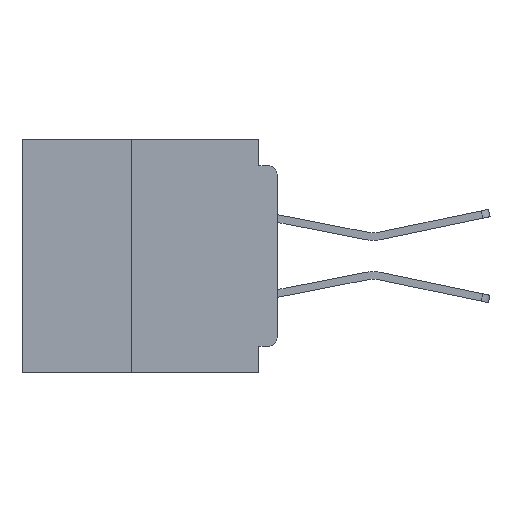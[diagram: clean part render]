
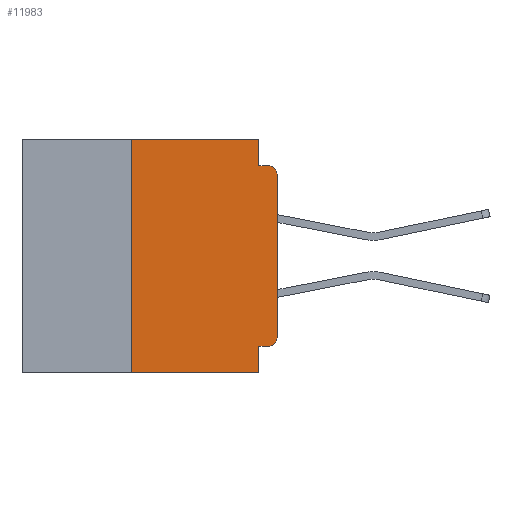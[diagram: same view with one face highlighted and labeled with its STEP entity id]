
A CAD part, left-side view. The second image highlights one B-rep face of the part: STEP entity #11983.
In plain terms, the highlighted planar face has unit normal (-1, 0, 0).
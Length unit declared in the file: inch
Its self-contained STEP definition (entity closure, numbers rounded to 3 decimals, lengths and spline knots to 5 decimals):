
#586 = DIRECTION ( 'NONE',  ( 0., 0., 1. ) ) ;
#776 = CARTESIAN_POINT ( 'NONE',  ( 0., 0.437, 0. ) ) ;
#959 = CARTESIAN_POINT ( 'NONE',  ( 0., 0.031, -0.4 ) ) ;
#1119 = LINE ( 'NONE', #18696, #9593 ) ;
#1357 = DIRECTION ( 'NONE',  ( 0., 0., -1. ) ) ;
#1956 = LINE ( 'NONE', #25080, #34847 ) ;
#2058 = LINE ( 'NONE', #19631, #9554 ) ;
#2086 = DIRECTION ( 'NONE',  ( -1., 0., 0. ) ) ;
#2098 = CARTESIAN_POINT ( 'NONE',  ( 0., 0.015, -0.06 ) ) ;
#2167 = CARTESIAN_POINT ( 'NONE',  ( 0., 0.015, -0.34 ) ) ;
#3313 = LINE ( 'NONE', #27133, #19255 ) ;
#3982 = PLANE ( 'NONE',  #41075 ) ;
#5369 = DIRECTION ( 'NONE',  ( 0., 0., -1. ) ) ;
#5922 = DIRECTION ( 'NONE',  ( 0., -1., 0. ) ) ;
#5979 = EDGE_CURVE ( 'NONE', #35043, #15358, #17767, .T. ) ;
#7226 = DIRECTION ( 'NONE',  ( 0., 0., -1. ) ) ;
#7338 = FACE_OUTER_BOUND ( 'NONE', #20604, .T. ) ;
#8306 = VERTEX_POINT ( 'NONE', #17071 ) ;
#8848 = ORIENTED_EDGE ( 'NONE', *, *, #27979, .F. ) ;
#9200 = DIRECTION ( 'NONE',  ( 0., 1., 0. ) ) ;
#9554 = VECTOR ( 'NONE', #586, 39.37008 ) ;
#9593 = VECTOR ( 'NONE', #34618, 39.37008 ) ;
#9607 = VERTEX_POINT ( 'NONE', #10606 ) ;
#9644 = VERTEX_POINT ( 'NONE', #13926 ) ;
#10606 = CARTESIAN_POINT ( 'NONE',  ( 0., 0., -0.34 ) ) ;
#11627 = EDGE_CURVE ( 'NONE', #9607, #35043, #3313, .T. ) ;
#11646 = CARTESIAN_POINT ( 'NONE',  ( 0., 0.437, -0.4 ) ) ;
#11672 = VERTEX_POINT ( 'NONE', #33660 ) ;
#11983 = ADVANCED_FACE ( 'NONE', ( #7338 ), #3982, .F. ) ;
#12351 = CARTESIAN_POINT ( 'NONE',  ( 0., 0., -0.045 ) ) ;
#12635 = CARTESIAN_POINT ( 'NONE',  ( 0., 0.031, -0.355 ) ) ;
#12803 = CARTESIAN_POINT ( 'NONE',  ( 0., 0.031, 0. ) ) ;
#12867 = LINE ( 'NONE', #31593, #28804 ) ;
#13926 = CARTESIAN_POINT ( 'NONE',  ( 0., 0.015, -0.355 ) ) ;
#14213 = EDGE_CURVE ( 'NONE', #32913, #32472, #1119, .T. ) ;
#14718 = CIRCLE ( 'NONE', #33610, 0.015 ) ;
#14750 = LINE ( 'NONE', #11646, #40142 ) ;
#15358 = VERTEX_POINT ( 'NONE', #18189 ) ;
#15528 = DIRECTION ( 'NONE',  ( 0., -1., 0. ) ) ;
#16445 = VECTOR ( 'NONE', #5922, 39.37008 ) ;
#16647 = EDGE_CURVE ( 'NONE', #9644, #32913, #1956, .T. ) ;
#17071 = CARTESIAN_POINT ( 'NONE',  ( 0., 0.031, -0.045 ) ) ;
#17425 = LINE ( 'NONE', #18552, #16445 ) ;
#17572 = ORIENTED_EDGE ( 'NONE', *, *, #11627, .T. ) ;
#17767 = CIRCLE ( 'NONE', #24394, 0.015 ) ;
#18125 = LINE ( 'NONE', #12351, #34094 ) ;
#18189 = CARTESIAN_POINT ( 'NONE',  ( 0., 0.015, -0.045 ) ) ;
#18446 = EDGE_CURVE ( 'NONE', #32080, #32472, #14750, .T. ) ;
#18552 = CARTESIAN_POINT ( 'NONE',  ( 0., 0.437, 0. ) ) ;
#18696 = CARTESIAN_POINT ( 'NONE',  ( 0., 0.031, -0.4 ) ) ;
#19194 = ORIENTED_EDGE ( 'NONE', *, *, #29186, .F. ) ;
#19255 = VECTOR ( 'NONE', #30341, 39.37008 ) ;
#19631 = CARTESIAN_POINT ( 'NONE',  ( 0., 0.25, -0.4 ) ) ;
#20580 = EDGE_CURVE ( 'NONE', #32080, #11672, #2058, .T. ) ;
#20604 = EDGE_LOOP ( 'NONE', ( #17572, #36741, #40418, #19194, #8848, #22691, #30998, #33156, #33685, #30481 ) ) ;
#22691 = ORIENTED_EDGE ( 'NONE', *, *, #20580, .F. ) ;
#24394 = AXIS2_PLACEMENT_3D ( 'NONE', #2098, #2086, #1357 ) ;
#24472 = DIRECTION ( 'NONE',  ( -1., 0., 0. ) ) ;
#25080 = CARTESIAN_POINT ( 'NONE',  ( 0., 0., -0.355 ) ) ;
#26274 = DIRECTION ( 'NONE',  ( 1., 0., 0. ) ) ;
#27133 = CARTESIAN_POINT ( 'NONE',  ( 0., 0., 0. ) ) ;
#27979 = EDGE_CURVE ( 'NONE', #11672, #31048, #17425, .T. ) ;
#28804 = VECTOR ( 'NONE', #34797, 39.37008 ) ;
#29186 = EDGE_CURVE ( 'NONE', #31048, #8306, #12867, .T. ) ;
#29598 = CARTESIAN_POINT ( 'NONE',  ( 0., 0., -0.06 ) ) ;
#30341 = DIRECTION ( 'NONE',  ( 0., 0., 1. ) ) ;
#30481 = ORIENTED_EDGE ( 'NONE', *, *, #38803, .T. ) ;
#30998 = ORIENTED_EDGE ( 'NONE', *, *, #18446, .T. ) ;
#31048 = VERTEX_POINT ( 'NONE', #12803 ) ;
#31593 = CARTESIAN_POINT ( 'NONE',  ( 0., 0.031, 0. ) ) ;
#31594 = EDGE_CURVE ( 'NONE', #8306, #15358, #18125, .T. ) ;
#32080 = VERTEX_POINT ( 'NONE', #33996 ) ;
#32472 = VERTEX_POINT ( 'NONE', #959 ) ;
#32913 = VERTEX_POINT ( 'NONE', #12635 ) ;
#33156 = ORIENTED_EDGE ( 'NONE', *, *, #14213, .F. ) ;
#33610 = AXIS2_PLACEMENT_3D ( 'NONE', #2167, #24472, #5369 ) ;
#33660 = CARTESIAN_POINT ( 'NONE',  ( 0., 0.25, 0. ) ) ;
#33685 = ORIENTED_EDGE ( 'NONE', *, *, #16647, .F. ) ;
#33895 = DIRECTION ( 'NONE',  ( 0., -1., 0. ) ) ;
#33996 = CARTESIAN_POINT ( 'NONE',  ( 0., 0.25, -0.4 ) ) ;
#34094 = VECTOR ( 'NONE', #15528, 39.37008 ) ;
#34618 = DIRECTION ( 'NONE',  ( 0., 0., -1. ) ) ;
#34797 = DIRECTION ( 'NONE',  ( 0., 0., -1. ) ) ;
#34847 = VECTOR ( 'NONE', #9200, 39.37008 ) ;
#35043 = VERTEX_POINT ( 'NONE', #29598 ) ;
#36741 = ORIENTED_EDGE ( 'NONE', *, *, #5979, .T. ) ;
#38803 = EDGE_CURVE ( 'NONE', #9644, #9607, #14718, .T. ) ;
#40142 = VECTOR ( 'NONE', #33895, 39.37008 ) ;
#40418 = ORIENTED_EDGE ( 'NONE', *, *, #31594, .F. ) ;
#41075 = AXIS2_PLACEMENT_3D ( 'NONE', #776, #26274, #7226 ) ;
